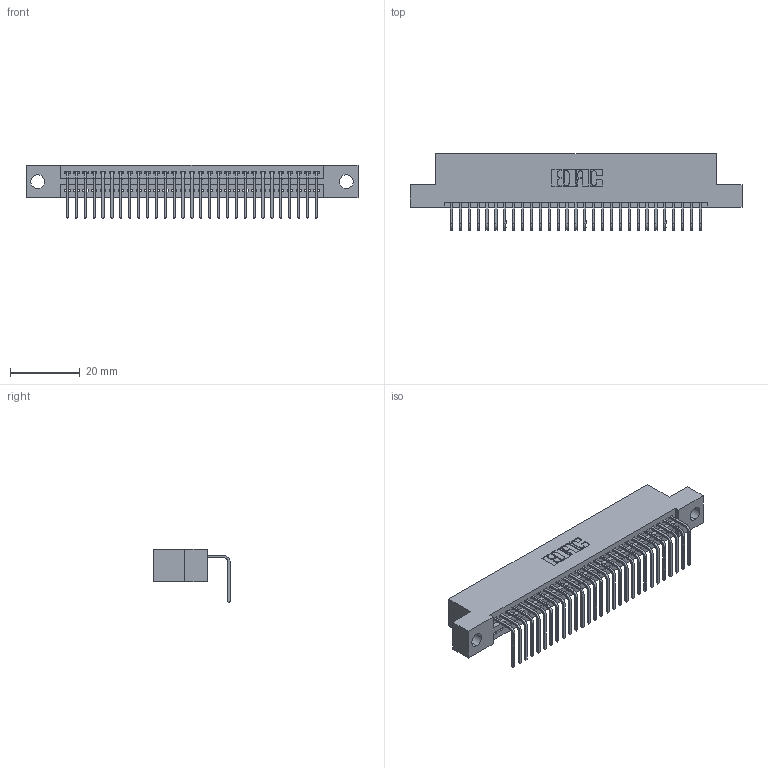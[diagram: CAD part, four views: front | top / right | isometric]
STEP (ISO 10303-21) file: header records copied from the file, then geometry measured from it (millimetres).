
FILE_DESCRIPTION (( 'STEP AP203' ), '1' );
FILE_NAME ('345-029-558-104.STEP', '2021-06-09T16:23:00', ( '' ), ( '' ), 'SwSTEP 2.0', 'SolidWorks 2020', '' );
FILE_SCHEMA (( 'CONFIG_CONTROL_DESIGN' ));
Length unit declared in the file: inch
Products named in the file (3): 345-029-558-104; 345-292-001_558 Tail - 2; 345 Part_Flush Mounting Lugs - 0.156 Dia-TI
Assembly tree (30 placements, depth 2):
  345-029-558-104
    345 Part_Flush Mounting Lugs - 0.156 Dia-TI
    345-292-001_558 Tail - 2  x29
Bounding box: 94.87 x 21.83 x 15.37 mm (x, y, z)
Volume: 8894.9 mm3; surface area: 12054.1 mm2
Topology: 30 solids, 30 shells, 1880 faces, 5655 edges, 3730 vertices
Faces by surface type: plane 1312, cylinder 568
Entity records: 24079 total; most frequent: CARTESIAN_POINT 4181, ORIENTED_EDGE 4142, DIRECTION 3669, EDGE_CURVE 2071, VECTOR 1823, LINE 1823, VERTEX_POINT 1378, AXIS2_PLACEMENT_3D 923
